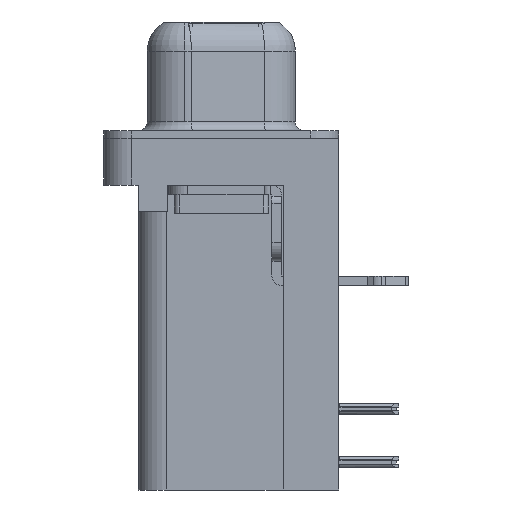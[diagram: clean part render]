
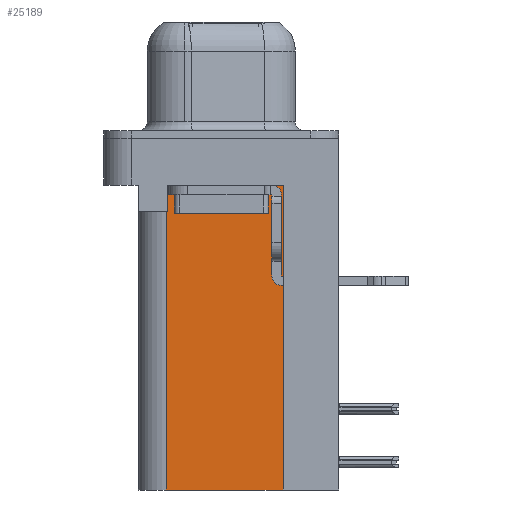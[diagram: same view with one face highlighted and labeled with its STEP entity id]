
A CAD part, left-side view. The second image highlights one B-rep face of the part: STEP entity #25189.
In plain terms, the highlighted planar face has unit normal (-1, 0, 0).
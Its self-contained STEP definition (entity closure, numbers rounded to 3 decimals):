
#945 = AXIS2_PLACEMENT_3D ( 'NONE', #12400, #1134, #20689 ) ;
#1134 = DIRECTION ( 'NONE',  ( 1., 0., 0. ) ) ;
#2019 = ORIENTED_EDGE ( 'NONE', *, *, #12212, .T. ) ;
#2386 = LINE ( 'NONE', #15389, #2436 ) ;
#2436 = VECTOR ( 'NONE', #20779, 1000. ) ;
#3228 = EDGE_CURVE ( 'NONE', #29301, #13348, #28737, .T. ) ;
#3274 = ORIENTED_EDGE ( 'NONE', *, *, #17374, .T. ) ;
#4596 = VERTEX_POINT ( 'NONE', #30889 ) ;
#5200 = VECTOR ( 'NONE', #30065, 1000. ) ;
#6452 = LINE ( 'NONE', #27464, #5200 ) ;
#6573 = LINE ( 'NONE', #31991, #7374 ) ;
#7374 = VECTOR ( 'NONE', #29620, 1000. ) ;
#9115 = ORIENTED_EDGE ( 'NONE', *, *, #3228, .T. ) ;
#10340 = VERTEX_POINT ( 'NONE', #22857 ) ;
#12212 = EDGE_CURVE ( 'NONE', #4596, #25484, #18578, .T. ) ;
#12400 = CARTESIAN_POINT ( 'NONE',  ( 3.79, -3.295, -18.76 ) ) ;
#13348 = VERTEX_POINT ( 'NONE', #32704 ) ;
#15389 = CARTESIAN_POINT ( 'NONE',  ( 3.79, -3.295, -18.76 ) ) ;
#16258 = CARTESIAN_POINT ( 'NONE',  ( 3.79, 2.895, -2.5 ) ) ;
#16679 = DIRECTION ( 'NONE',  ( 0., 1., 0. ) ) ;
#17374 = EDGE_CURVE ( 'NONE', #25484, #29301, #34297, .T. ) ;
#17986 = PLANE ( 'NONE',  #945 ) ;
#18239 = CARTESIAN_POINT ( 'NONE',  ( 3.79, 2.895, -3.9 ) ) ;
#18578 = LINE ( 'NONE', #29713, #18644 ) ;
#18644 = VECTOR ( 'NONE', #16679, 1000. ) ;
#19630 = ORIENTED_EDGE ( 'NONE', *, *, #31680, .F. ) ;
#20666 = CARTESIAN_POINT ( 'NONE',  ( 3.79, 2.925, -18.76 ) ) ;
#20689 = DIRECTION ( 'NONE',  ( 0., 1., 0. ) ) ;
#20779 = DIRECTION ( 'NONE',  ( 0., 1., 0. ) ) ;
#21049 = DIRECTION ( 'NONE',  ( 0., 0., -1. ) ) ;
#21809 = CARTESIAN_POINT ( 'NONE',  ( 3.79, 0., -3.9 ) ) ;
#22089 = FACE_OUTER_BOUND ( 'NONE', #30685, .T. ) ;
#22857 = CARTESIAN_POINT ( 'NONE',  ( 3.79, -3.295, -18.76 ) ) ;
#23901 = CARTESIAN_POINT ( 'NONE',  ( 3.79, 2.895, -3.9 ) ) ;
#25189 = ADVANCED_FACE ( 'NONE', ( #22089 ), #17986, .F. ) ;
#25484 = VERTEX_POINT ( 'NONE', #16258 ) ;
#25790 = ORIENTED_EDGE ( 'NONE', *, *, #31863, .T. ) ;
#27464 = CARTESIAN_POINT ( 'NONE',  ( 3.79, -3.295, -18.76 ) ) ;
#27886 = ORIENTED_EDGE ( 'NONE', *, *, #29137, .F. ) ;
#28737 = LINE ( 'NONE', #21809, #28845 ) ;
#28845 = VECTOR ( 'NONE', #29281, 1000. ) ;
#29137 = EDGE_CURVE ( 'NONE', #10340, #32714, #2386, .T. ) ;
#29281 = DIRECTION ( 'NONE',  ( 0., 1., 0. ) ) ;
#29301 = VERTEX_POINT ( 'NONE', #23901 ) ;
#29620 = DIRECTION ( 'NONE',  ( 0., 0., 1. ) ) ;
#29713 = CARTESIAN_POINT ( 'NONE',  ( 3.79, -3.295, -2.5 ) ) ;
#30065 = DIRECTION ( 'NONE',  ( 0., 0., 1. ) ) ;
#30685 = EDGE_LOOP ( 'NONE', ( #2019, #3274, #9115, #19630, #27886, #25790 ) ) ;
#30889 = CARTESIAN_POINT ( 'NONE',  ( 3.79, -3.295, -2.5 ) ) ;
#31680 = EDGE_CURVE ( 'NONE', #32714, #13348, #6573, .T. ) ;
#31863 = EDGE_CURVE ( 'NONE', #10340, #4596, #6452, .T. ) ;
#31991 = CARTESIAN_POINT ( 'NONE',  ( 3.79, 2.925, -18.76 ) ) ;
#32704 = CARTESIAN_POINT ( 'NONE',  ( 3.79, 2.925, -3.9 ) ) ;
#32714 = VERTEX_POINT ( 'NONE', #20666 ) ;
#34268 = VECTOR ( 'NONE', #21049, 1000. ) ;
#34297 = LINE ( 'NONE', #18239, #34268 ) ;
